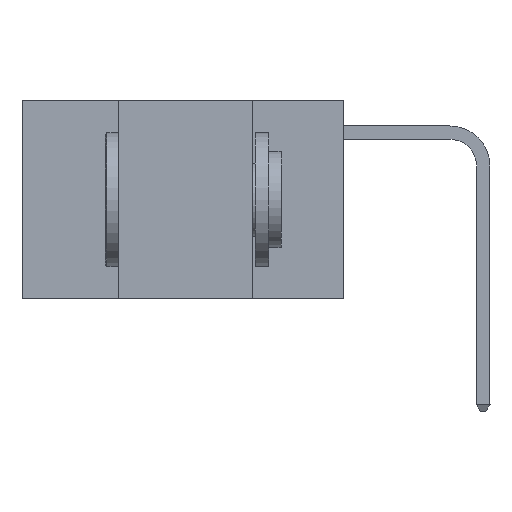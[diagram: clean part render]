
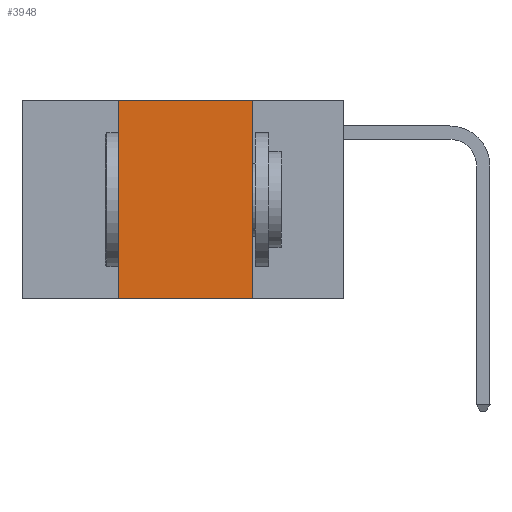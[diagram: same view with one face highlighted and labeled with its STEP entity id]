
A CAD part, left-side view. The second image highlights one B-rep face of the part: STEP entity #3948.
In plain terms, the highlighted planar face has unit normal (-1, 0, 0).
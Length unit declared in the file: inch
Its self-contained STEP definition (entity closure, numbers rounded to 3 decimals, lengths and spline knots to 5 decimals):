
#420 = CARTESIAN_POINT ( 'NONE',  ( 0., 0.6, -0.37 ) ) ;
#859 = DIRECTION ( 'NONE',  ( 1., 0., 0. ) ) ;
#1368 = AXIS2_PLACEMENT_3D ( 'NONE', #24007, #859, #17028 ) ;
#2014 = ORIENTED_EDGE ( 'NONE', *, *, #6509, .F. ) ;
#2619 = DIRECTION ( 'NONE',  ( 0., -1., 0. ) ) ;
#2963 = CARTESIAN_POINT ( 'NONE',  ( 0., 0.42, 0. ) ) ;
#3948 = ADVANCED_FACE ( 'NONE', ( #25803 ), #28454, .F. ) ;
#4255 = CARTESIAN_POINT ( 'NONE',  ( 0., 0.6, 0. ) ) ;
#4855 = CARTESIAN_POINT ( 'NONE',  ( 0., 0.42, 0. ) ) ;
#6024 = DIRECTION ( 'NONE',  ( 0., 0., -1. ) ) ;
#6509 = EDGE_CURVE ( 'NONE', #11845, #15061, #9812, .T. ) ;
#7242 = LINE ( 'NONE', #420, #19466 ) ;
#7667 = LINE ( 'NONE', #25936, #14580 ) ;
#9812 = LINE ( 'NONE', #2963, #26727 ) ;
#10966 = CARTESIAN_POINT ( 'NONE',  ( 0., 0.42, -0.37 ) ) ;
#11126 = ORIENTED_EDGE ( 'NONE', *, *, #23657, .F. ) ;
#11845 = VERTEX_POINT ( 'NONE', #10966 ) ;
#12523 = ORIENTED_EDGE ( 'NONE', *, *, #16433, .T. ) ;
#12803 = VECTOR ( 'NONE', #15124, 39.37008 ) ;
#14580 = VECTOR ( 'NONE', #6024, 39.37008 ) ;
#15061 = VERTEX_POINT ( 'NONE', #4855 ) ;
#15124 = DIRECTION ( 'NONE',  ( 0., -1., 0. ) ) ;
#16433 = EDGE_CURVE ( 'NONE', #11845, #28646, #7242, .T. ) ;
#17028 = DIRECTION ( 'NONE',  ( 0., 0., -1. ) ) ;
#17990 = EDGE_LOOP ( 'NONE', ( #24021, #11126, #2014, #12523 ) ) ;
#18570 = VERTEX_POINT ( 'NONE', #23931 ) ;
#19437 = EDGE_CURVE ( 'NONE', #18570, #28646, #7667, .T. ) ;
#19466 = VECTOR ( 'NONE', #2619, 39.37008 ) ;
#20585 = CARTESIAN_POINT ( 'NONE',  ( 0., 0.17, -0.37 ) ) ;
#23657 = EDGE_CURVE ( 'NONE', #15061, #18570, #24027, .T. ) ;
#23931 = CARTESIAN_POINT ( 'NONE',  ( 0., 0.17, 0. ) ) ;
#24007 = CARTESIAN_POINT ( 'NONE',  ( 0., 0.6, 0. ) ) ;
#24021 = ORIENTED_EDGE ( 'NONE', *, *, #19437, .F. ) ;
#24027 = LINE ( 'NONE', #4255, #12803 ) ;
#25803 = FACE_OUTER_BOUND ( 'NONE', #17990, .T. ) ;
#25936 = CARTESIAN_POINT ( 'NONE',  ( 0., 0.17, 0. ) ) ;
#26727 = VECTOR ( 'NONE', #28752, 39.37008 ) ;
#28454 = PLANE ( 'NONE',  #1368 ) ;
#28646 = VERTEX_POINT ( 'NONE', #20585 ) ;
#28752 = DIRECTION ( 'NONE',  ( 0., 0., 1. ) ) ;
